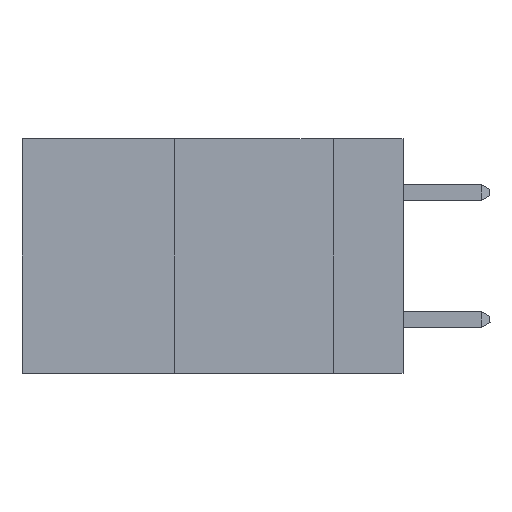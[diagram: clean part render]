
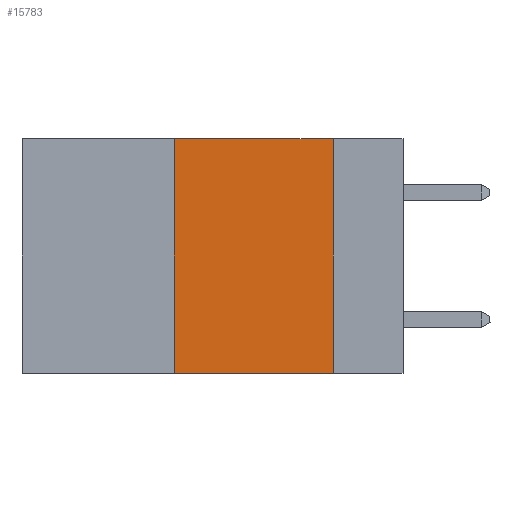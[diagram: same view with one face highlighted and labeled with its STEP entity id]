
A CAD part, left-side view. The second image highlights one B-rep face of the part: STEP entity #15783.
In plain terms, the highlighted planar face has unit normal (-1, 0, 0).
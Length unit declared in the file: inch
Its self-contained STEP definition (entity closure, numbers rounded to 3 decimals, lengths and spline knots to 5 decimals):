
#216 = CARTESIAN_POINT ( 'NONE',  ( 0., 0.36, 0. ) ) ;
#315 = LINE ( 'NONE', #14338, #13479 ) ;
#481 = EDGE_CURVE ( 'NONE', #14424, #2849, #315, .T. ) ;
#651 = CARTESIAN_POINT ( 'NONE',  ( 0., 0.6, 0. ) ) ;
#1230 = DIRECTION ( 'NONE',  ( 1., 0., 0. ) ) ;
#1641 = VERTEX_POINT ( 'NONE', #16384 ) ;
#1682 = CARTESIAN_POINT ( 'NONE',  ( 0., 0.11, -0.37 ) ) ;
#2222 = LINE ( 'NONE', #651, #20614 ) ;
#2849 = VERTEX_POINT ( 'NONE', #216 ) ;
#5332 = VERTEX_POINT ( 'NONE', #1682 ) ;
#6312 = VECTOR ( 'NONE', #9227, 39.37008 ) ;
#6481 = FACE_OUTER_BOUND ( 'NONE', #6985, .T. ) ;
#6718 = EDGE_CURVE ( 'NONE', #14424, #5332, #15700, .T. ) ;
#6985 = EDGE_LOOP ( 'NONE', ( #8380, #15866, #17251, #16653 ) ) ;
#7252 = DIRECTION ( 'NONE',  ( 0., 0., 1. ) ) ;
#8380 = ORIENTED_EDGE ( 'NONE', *, *, #15109, .F. ) ;
#9227 = DIRECTION ( 'NONE',  ( 0., -1., 0. ) ) ;
#9324 = DIRECTION ( 'NONE',  ( 0., -1., 0. ) ) ;
#10403 = EDGE_CURVE ( 'NONE', #2849, #1641, #2222, .T. ) ;
#10906 = LINE ( 'NONE', #20900, #20905 ) ;
#13479 = VECTOR ( 'NONE', #7252, 39.37008 ) ;
#13710 = DIRECTION ( 'NONE',  ( 0., 0., -1. ) ) ;
#14338 = CARTESIAN_POINT ( 'NONE',  ( 0., 0.36, 0. ) ) ;
#14424 = VERTEX_POINT ( 'NONE', #17177 ) ;
#15109 = EDGE_CURVE ( 'NONE', #1641, #5332, #10906, .T. ) ;
#15700 = LINE ( 'NONE', #18024, #6312 ) ;
#15783 = ADVANCED_FACE ( 'NONE', ( #6481 ), #22577, .F. ) ;
#15866 = ORIENTED_EDGE ( 'NONE', *, *, #10403, .F. ) ;
#16384 = CARTESIAN_POINT ( 'NONE',  ( 0., 0.11, 0. ) ) ;
#16653 = ORIENTED_EDGE ( 'NONE', *, *, #6718, .T. ) ;
#17177 = CARTESIAN_POINT ( 'NONE',  ( 0., 0.36, -0.37 ) ) ;
#17251 = ORIENTED_EDGE ( 'NONE', *, *, #481, .F. ) ;
#18024 = CARTESIAN_POINT ( 'NONE',  ( 0., 0.6, -0.37 ) ) ;
#18989 = CARTESIAN_POINT ( 'NONE',  ( 0., 0.6, 0. ) ) ;
#19097 = DIRECTION ( 'NONE',  ( 0., 0., -1. ) ) ;
#20614 = VECTOR ( 'NONE', #9324, 39.37008 ) ;
#20900 = CARTESIAN_POINT ( 'NONE',  ( 0., 0.11, 0. ) ) ;
#20905 = VECTOR ( 'NONE', #19097, 39.37008 ) ;
#21415 = AXIS2_PLACEMENT_3D ( 'NONE', #18989, #1230, #13710 ) ;
#22577 = PLANE ( 'NONE',  #21415 ) ;
